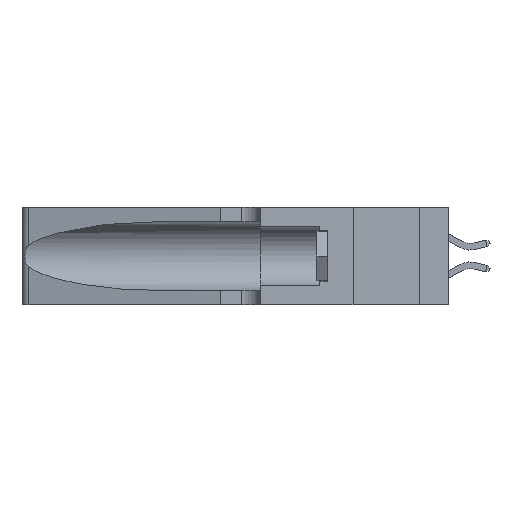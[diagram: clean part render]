
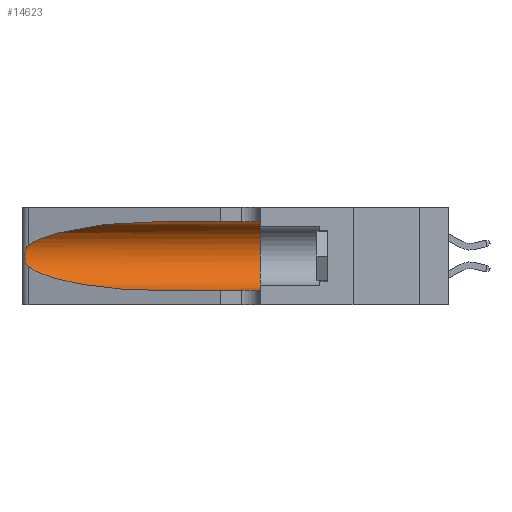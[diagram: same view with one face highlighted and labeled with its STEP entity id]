
A CAD part, left-side view. The second image highlights one B-rep face of the part: STEP entity #14623.
In plain terms, the highlighted cylindrical face has radius 3.308 mm (diameter 6.617 mm), a partial arc.
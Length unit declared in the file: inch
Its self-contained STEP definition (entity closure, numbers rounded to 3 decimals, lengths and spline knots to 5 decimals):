
#145 = CARTESIAN_POINT ( 'NONE',  ( 0.26075, 1.23896, 0.178 ) ) ;
#479 = CARTESIAN_POINT ( 'NONE',  ( 0.26075, 1.23896, 0.19203 ) ) ;
#909 = CARTESIAN_POINT ( 'NONE',  ( 0.25487, 1.22718, 0.14631 ) ) ;
#996 = CARTESIAN_POINT ( 'NONE',  ( 0.25487, 1.22718, 0.22369 ) ) ;
#1019 = AXIS2_PLACEMENT_3D ( 'NONE', #13750, #2462, #19259 ) ;
#1134 = ORIENTED_EDGE ( 'NONE', *, *, #18471, .T. ) ;
#1455 = EDGE_CURVE ( 'NONE', #13644, #14337, #7541, .T. ) ;
#1581 = CARTESIAN_POINT ( 'NONE',  ( 0.2373, 1.15595, 0.28018 ) ) ;
#2462 = DIRECTION ( 'NONE',  ( 0., -1., 0. ) ) ;
#3027 = CARTESIAN_POINT ( 'NONE',  ( 0.1305, 0.35, 0.05475 ) ) ;
#3528 = ORIENTED_EDGE ( 'NONE', *, *, #15578, .F. ) ;
#4952 = EDGE_CURVE ( 'NONE', #14337, #19070, #23259, .T. ) ;
#5266 = B_SPLINE_CURVE_WITH_KNOTS ( 'NONE', 3,
 ( #11812, #21093, #7718, #22727, #5955, #11727, #479, #145, #19305, #8046, #21176, #13385, #9911, #23060 ),
 .UNSPECIFIED., .F., .F.,
 ( 4, 2, 2, 2, 2, 2, 4 ),
 ( 0., 0.00027, 0.00053, 0.00107, 0.0016, 0.00187, 0.00214 ),
 .UNSPECIFIED. ) ;
#5955 = CARTESIAN_POINT ( 'NONE',  ( 0.25854, 1.2359, 0.20912 ) ) ;
#6279 = CARTESIAN_POINT ( 'NONE',  ( 0.2373, 1.15595, 0.08982 ) ) ;
#6732 = DIRECTION ( 'NONE',  ( 0., -1., 0. ) ) ;
#6756 = VERTEX_POINT ( 'NONE', #23105 ) ;
#7048 = ORIENTED_EDGE ( 'NONE', *, *, #20375, .F. ) ;
#7541 =( BOUNDED_CURVE ( )  B_SPLINE_CURVE ( 3, ( #909, #6279, #21567, #23391 ),
 .UNSPECIFIED., .F., .F. ) 
 B_SPLINE_CURVE_WITH_KNOTS ( ( 4, 4 ),
 ( 3.44316, 4.71239 ),
 .UNSPECIFIED. ) 
 CURVE ( )  GEOMETRIC_REPRESENTATION_ITEM ( )  RATIONAL_B_SPLINE_CURVE ( ( 1., 0.87, 0.87, 1. ) ) 
 REPRESENTATION_ITEM ( '' )  );
#7718 = CARTESIAN_POINT ( 'NONE',  ( 0.25639, 1.23184, 0.21858 ) ) ;
#7960 = CARTESIAN_POINT ( 'NONE',  ( 0.1305, 1.61858, 0.31525 ) ) ;
#8046 = CARTESIAN_POINT ( 'NONE',  ( 0.25856, 1.23593, 0.16098 ) ) ;
#9045 = DIRECTION ( 'NONE',  ( 0., 0., 1. ) ) ;
#9137 = FACE_OUTER_BOUND ( 'NONE', #17853, .T. ) ;
#9335 =( BOUNDED_CURVE ( )  B_SPLINE_CURVE ( 3, ( #22459, #13052, #1581, #16766 ),
 .UNSPECIFIED., .F., .F. ) 
 B_SPLINE_CURVE_WITH_KNOTS ( ( 4, 4 ),
 ( 1.5708, 2.84003 ),
 .UNSPECIFIED. ) 
 CURVE ( )  GEOMETRIC_REPRESENTATION_ITEM ( )  RATIONAL_B_SPLINE_CURVE ( ( 1., 0.87, 0.87, 1. ) ) 
 REPRESENTATION_ITEM ( '' )  );
#9911 = CARTESIAN_POINT ( 'NONE',  ( 0.25555, 1.22993, 0.14849 ) ) ;
#10055 = VERTEX_POINT ( 'NONE', #996 ) ;
#10447 = CARTESIAN_POINT ( 'NONE',  ( 0.1305, 0.72297, 0.05475 ) ) ;
#10762 = DIRECTION ( 'NONE',  ( 0., 1., 0. ) ) ;
#10837 = ORIENTED_EDGE ( 'NONE', *, *, #4952, .T. ) ;
#11163 = CIRCLE ( 'NONE', #23738, 0.13025 ) ;
#11726 = ORIENTED_EDGE ( 'NONE', *, *, #19256, .T. ) ;
#11727 = CARTESIAN_POINT ( 'NONE',  ( 0.26018, 1.23835, 0.19895 ) ) ;
#11812 = CARTESIAN_POINT ( 'NONE',  ( 0.25487, 1.22718, 0.22369 ) ) ;
#12363 = DIRECTION ( 'NONE',  ( 0., -1., 0. ) ) ;
#12973 = CYLINDRICAL_SURFACE ( 'NONE', #1019, 0.13025 ) ;
#13052 = CARTESIAN_POINT ( 'NONE',  ( 0.18966, 0.96281, 0.31525 ) ) ;
#13385 = CARTESIAN_POINT ( 'NONE',  ( 0.25639, 1.23186, 0.15144 ) ) ;
#13644 = VERTEX_POINT ( 'NONE', #23153 ) ;
#13750 = CARTESIAN_POINT ( 'NONE',  ( 0.1305, 1.61858, 0.185 ) ) ;
#14337 = VERTEX_POINT ( 'NONE', #10447 ) ;
#14623 = ADVANCED_FACE ( 'NONE', ( #9137 ), #12973, .F. ) ;
#15578 = EDGE_CURVE ( 'NONE', #6756, #19070, #11163, .T. ) ;
#16766 = CARTESIAN_POINT ( 'NONE',  ( 0.25487, 1.22718, 0.22369 ) ) ;
#17853 = EDGE_LOOP ( 'NONE', ( #1134, #11726, #21060, #10837, #3528, #7048 ) ) ;
#18022 = CARTESIAN_POINT ( 'NONE',  ( 0.1305, 1.61858, 0.05475 ) ) ;
#18471 = EDGE_CURVE ( 'NONE', #19036, #10055, #9335, .T. ) ;
#19036 = VERTEX_POINT ( 'NONE', #21121 ) ;
#19070 = VERTEX_POINT ( 'NONE', #3027 ) ;
#19256 = EDGE_CURVE ( 'NONE', #10055, #13644, #5266, .T. ) ;
#19259 = DIRECTION ( 'NONE',  ( 0., 0., -1. ) ) ;
#19305 = CARTESIAN_POINT ( 'NONE',  ( 0.26017, 1.23833, 0.17102 ) ) ;
#20317 = VECTOR ( 'NONE', #6732, 39.37008 ) ;
#20375 = EDGE_CURVE ( 'NONE', #19036, #6756, #23325, .T. ) ;
#21060 = ORIENTED_EDGE ( 'NONE', *, *, #1455, .T. ) ;
#21093 = CARTESIAN_POINT ( 'NONE',  ( 0.25555, 1.22994, 0.2215 ) ) ;
#21121 = CARTESIAN_POINT ( 'NONE',  ( 0.1305, 0.72297, 0.31525 ) ) ;
#21176 = CARTESIAN_POINT ( 'NONE',  ( 0.25789, 1.23486, 0.15765 ) ) ;
#21567 = CARTESIAN_POINT ( 'NONE',  ( 0.18966, 0.96281, 0.05475 ) ) ;
#22459 = CARTESIAN_POINT ( 'NONE',  ( 0.1305, 0.72297, 0.31525 ) ) ;
#22727 = CARTESIAN_POINT ( 'NONE',  ( 0.25787, 1.23484, 0.2124 ) ) ;
#23060 = CARTESIAN_POINT ( 'NONE',  ( 0.25487, 1.22718, 0.14631 ) ) ;
#23105 = CARTESIAN_POINT ( 'NONE',  ( 0.1305, 0.35, 0.31525 ) ) ;
#23153 = CARTESIAN_POINT ( 'NONE',  ( 0.25487, 1.22718, 0.14631 ) ) ;
#23259 = LINE ( 'NONE', #18022, #20317 ) ;
#23325 = LINE ( 'NONE', #7960, #24199 ) ;
#23391 = CARTESIAN_POINT ( 'NONE',  ( 0.1305, 0.72297, 0.05475 ) ) ;
#23738 = AXIS2_PLACEMENT_3D ( 'NONE', #24085, #10762, #9045 ) ;
#24085 = CARTESIAN_POINT ( 'NONE',  ( 0.1305, 0.35, 0.185 ) ) ;
#24199 = VECTOR ( 'NONE', #12363, 39.37008 ) ;
